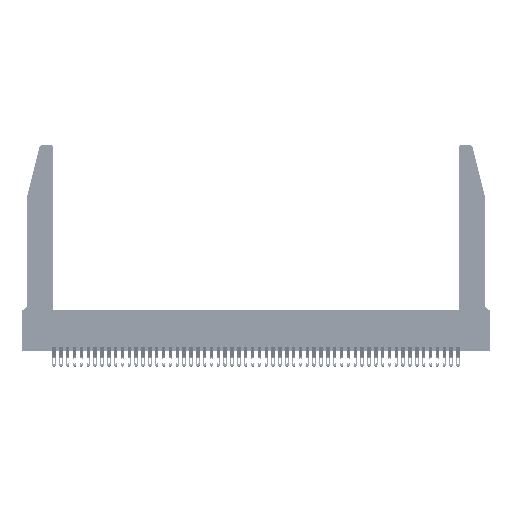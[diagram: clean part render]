
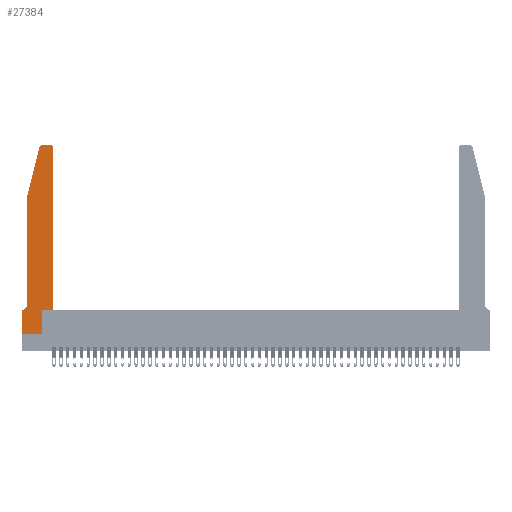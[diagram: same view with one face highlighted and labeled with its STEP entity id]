
A CAD part, top view. The second image highlights one B-rep face of the part: STEP entity #27384.
In plain terms, the highlighted planar face has unit normal (0, 0, 1).
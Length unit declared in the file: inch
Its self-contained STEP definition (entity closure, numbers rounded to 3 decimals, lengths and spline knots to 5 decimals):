
#566 = ORIENTED_EDGE ( 'NONE', *, *, #18215, .T. ) ;
#1000 = EDGE_CURVE ( 'NONE', #23278, #26579, #33402, .T. ) ;
#1257 = DIRECTION ( 'NONE',  ( 1., 0., 0. ) ) ;
#1468 = LINE ( 'NONE', #24098, #13057 ) ;
#3666 = LINE ( 'NONE', #24473, #20682 ) ;
#3678 = CARTESIAN_POINT ( 'NONE',  ( 0.4205, 2.75, 0.37 ) ) ;
#4088 = VERTEX_POINT ( 'NONE', #3678 ) ;
#4210 = CARTESIAN_POINT ( 'NONE',  ( 0.4505, 0.35, 0.37 ) ) ;
#4367 = CARTESIAN_POINT ( 'NONE',  ( 0.0755, 0.42, 0.37 ) ) ;
#5957 = DIRECTION ( 'NONE',  ( 0., 1., 0. ) ) ;
#6188 = EDGE_CURVE ( 'NONE', #12513, #23278, #28792, .T. ) ;
#6657 = CARTESIAN_POINT ( 'NONE',  ( 0.0755, 0.35, 0.37 ) ) ;
#7507 = DIRECTION ( 'NONE',  ( -0.239, -0.971, 0. ) ) ;
#7933 = VECTOR ( 'NONE', #7507, 39.37008 ) ;
#8755 = CIRCLE ( 'NONE', #17522, 0.03 ) ;
#10006 = EDGE_LOOP ( 'NONE', ( #39338, #13142, #26735, #23117, #35399, #48562, #31720, #566, #22150, #31806, #11989, #39117 ) ) ;
#10548 = DIRECTION ( 'NONE',  ( -1., 0., 0. ) ) ;
#10684 = CARTESIAN_POINT ( 'NONE',  ( 0.284, 2.72, 0.37 ) ) ;
#11235 = CARTESIAN_POINT ( 'NONE',  ( 0.0755, 2., 0.37 ) ) ;
#11644 = CARTESIAN_POINT ( 'NONE',  ( 0.4505, 0.35, 0.37 ) ) ;
#11804 = CARTESIAN_POINT ( 'NONE',  ( 0., 0.35, 0.37 ) ) ;
#11989 = ORIENTED_EDGE ( 'NONE', *, *, #29101, .T. ) ;
#12502 = CARTESIAN_POINT ( 'NONE',  ( 0.2865, 0., 0.37 ) ) ;
#12513 = VERTEX_POINT ( 'NONE', #4367 ) ;
#12521 = LINE ( 'NONE', #44268, #20388 ) ;
#12784 = CARTESIAN_POINT ( 'NONE',  ( 0.2605, 2.75, 0.37 ) ) ;
#13057 = VECTOR ( 'NONE', #31960, 39.37008 ) ;
#13142 = ORIENTED_EDGE ( 'NONE', *, *, #34832, .T. ) ;
#13759 = CARTESIAN_POINT ( 'NONE',  ( 0., 0., 0.37 ) ) ;
#13780 = VERTEX_POINT ( 'NONE', #20218 ) ;
#14232 = VERTEX_POINT ( 'NONE', #29094 ) ;
#14605 = DIRECTION ( 'NONE',  ( 1., 0., 0. ) ) ;
#15036 = VERTEX_POINT ( 'NONE', #25848 ) ;
#15410 = VERTEX_POINT ( 'NONE', #12502 ) ;
#15429 = EDGE_CURVE ( 'NONE', #13780, #4088, #34066, .T. ) ;
#16408 = LINE ( 'NONE', #12784, #45687 ) ;
#16429 = AXIS2_PLACEMENT_3D ( 'NONE', #17269, #44010, #21153 ) ;
#17269 = CARTESIAN_POINT ( 'NONE',  ( 0.0055, 0.42, 0.37 ) ) ;
#17522 = AXIS2_PLACEMENT_3D ( 'NONE', #10684, #37567, #14605 ) ;
#17584 = DIRECTION ( 'NONE',  ( 0., 1., 0. ) ) ;
#17666 = CARTESIAN_POINT ( 'NONE',  ( 0.2865, 0.35, 0.37 ) ) ;
#18215 = EDGE_CURVE ( 'NONE', #49559, #15410, #3666, .T. ) ;
#18962 = VERTEX_POINT ( 'NONE', #17666 ) ;
#19320 = EDGE_CURVE ( 'NONE', #18962, #43024, #23568, .T. ) ;
#19572 = PLANE ( 'NONE',  #36873 ) ;
#20218 = CARTESIAN_POINT ( 'NONE',  ( 0.4505, 2.72, 0.37 ) ) ;
#20388 = VECTOR ( 'NONE', #5957, 39.37008 ) ;
#20452 = DIRECTION ( 'NONE',  ( 0., 0., 1. ) ) ;
#20682 = VECTOR ( 'NONE', #1257, 39.37008 ) ;
#21153 = DIRECTION ( 'NONE',  ( -1., 0., 0. ) ) ;
#22150 = ORIENTED_EDGE ( 'NONE', *, *, #46332, .T. ) ;
#22732 = CARTESIAN_POINT ( 'NONE',  ( 0., 0., 0.37 ) ) ;
#23117 = ORIENTED_EDGE ( 'NONE', *, *, #34519, .T. ) ;
#23278 = VERTEX_POINT ( 'NONE', #27953 ) ;
#23470 = DIRECTION ( 'NONE',  ( 1., 0., 0. ) ) ;
#23525 = FACE_OUTER_BOUND ( 'NONE', #10006, .T. ) ;
#23568 = LINE ( 'NONE', #4210, #32551 ) ;
#24098 = CARTESIAN_POINT ( 'NONE',  ( 0.0755, 2., 0.37 ) ) ;
#24473 = CARTESIAN_POINT ( 'NONE',  ( 0., 0., 0.37 ) ) ;
#25848 = CARTESIAN_POINT ( 'NONE',  ( 0.25487, 2.72718, 0.37 ) ) ;
#26579 = VERTEX_POINT ( 'NONE', #30228 ) ;
#26735 = ORIENTED_EDGE ( 'NONE', *, *, #32342, .T. ) ;
#27292 = LINE ( 'NONE', #11235, #7933 ) ;
#27384 = ADVANCED_FACE ( 'NONE', ( #23525 ), #19572, .T. ) ;
#27477 = VERTEX_POINT ( 'NONE', #39306 ) ;
#27953 = CARTESIAN_POINT ( 'NONE',  ( 0.0055, 0.35, 0.37 ) ) ;
#28792 = CIRCLE ( 'NONE', #16429, 0.07 ) ;
#29094 = CARTESIAN_POINT ( 'NONE',  ( 0.284, 2.75, 0.37 ) ) ;
#29101 = EDGE_CURVE ( 'NONE', #43024, #13780, #48395, .T. ) ;
#29706 = LINE ( 'NONE', #22732, #39835 ) ;
#30228 = CARTESIAN_POINT ( 'NONE',  ( 0., 0.35, 0.37 ) ) ;
#31720 = ORIENTED_EDGE ( 'NONE', *, *, #36444, .T. ) ;
#31806 = ORIENTED_EDGE ( 'NONE', *, *, #19320, .T. ) ;
#31960 = DIRECTION ( 'NONE',  ( 0., -1., 0. ) ) ;
#32342 = EDGE_CURVE ( 'NONE', #15036, #27477, #27292, .T. ) ;
#32551 = VECTOR ( 'NONE', #46382, 39.37008 ) ;
#33402 = LINE ( 'NONE', #6657, #41129 ) ;
#34066 = CIRCLE ( 'NONE', #46136, 0.03 ) ;
#34519 = EDGE_CURVE ( 'NONE', #27477, #12513, #1468, .T. ) ;
#34832 = EDGE_CURVE ( 'NONE', #14232, #15036, #8755, .T. ) ;
#35399 = ORIENTED_EDGE ( 'NONE', *, *, #6188, .T. ) ;
#35789 = DIRECTION ( 'NONE',  ( -1., 0., 0. ) ) ;
#36444 = EDGE_CURVE ( 'NONE', #26579, #49559, #29706, .T. ) ;
#36668 = CARTESIAN_POINT ( 'NONE',  ( 0.4505, 0.35, 0.37 ) ) ;
#36873 = AXIS2_PLACEMENT_3D ( 'NONE', #11804, #46306, #23470 ) ;
#37567 = DIRECTION ( 'NONE',  ( 0., 0., 1. ) ) ;
#37967 = EDGE_CURVE ( 'NONE', #4088, #14232, #16408, .T. ) ;
#38277 = VECTOR ( 'NONE', #17584, 39.37008 ) ;
#39117 = ORIENTED_EDGE ( 'NONE', *, *, #15429, .T. ) ;
#39306 = CARTESIAN_POINT ( 'NONE',  ( 0.0755, 2., 0.37 ) ) ;
#39338 = ORIENTED_EDGE ( 'NONE', *, *, #37967, .T. ) ;
#39835 = VECTOR ( 'NONE', #45733, 39.37008 ) ;
#41129 = VECTOR ( 'NONE', #10548, 39.37008 ) ;
#43024 = VERTEX_POINT ( 'NONE', #11644 ) ;
#43323 = CARTESIAN_POINT ( 'NONE',  ( 0.4205, 2.72, 0.37 ) ) ;
#44010 = DIRECTION ( 'NONE',  ( 0., 0., -1. ) ) ;
#44268 = CARTESIAN_POINT ( 'NONE',  ( 0.2865, 0.35, 0.37 ) ) ;
#45687 = VECTOR ( 'NONE', #35789, 39.37008 ) ;
#45733 = DIRECTION ( 'NONE',  ( 0., -1., 0. ) ) ;
#46136 = AXIS2_PLACEMENT_3D ( 'NONE', #43323, #20452, #47145 ) ;
#46306 = DIRECTION ( 'NONE',  ( 0., 0., 1. ) ) ;
#46332 = EDGE_CURVE ( 'NONE', #15410, #18962, #12521, .T. ) ;
#46382 = DIRECTION ( 'NONE',  ( 1., 0., 0. ) ) ;
#47145 = DIRECTION ( 'NONE',  ( 1., 0., 0. ) ) ;
#48395 = LINE ( 'NONE', #36668, #38277 ) ;
#48562 = ORIENTED_EDGE ( 'NONE', *, *, #1000, .T. ) ;
#49559 = VERTEX_POINT ( 'NONE', #13759 ) ;
